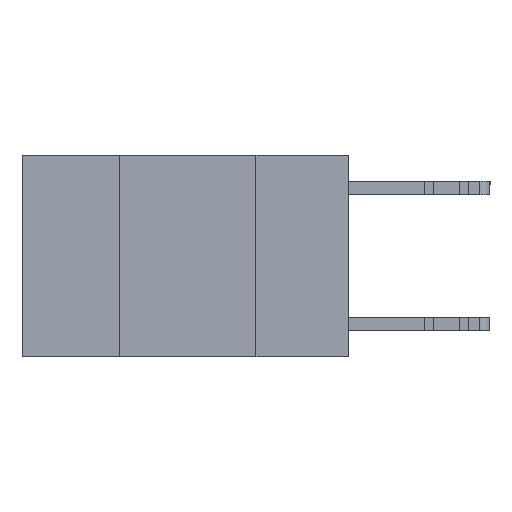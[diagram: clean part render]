
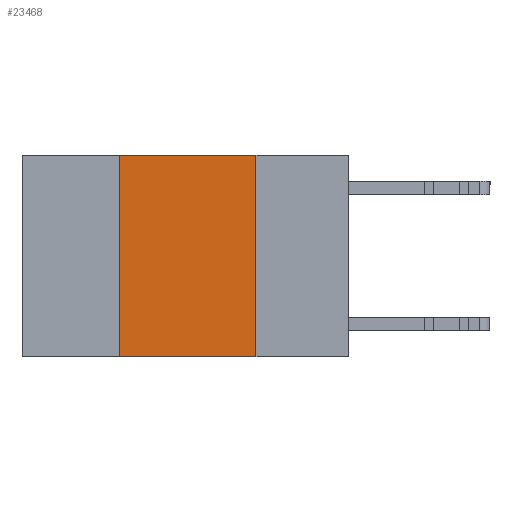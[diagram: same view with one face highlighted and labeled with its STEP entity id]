
A CAD part, left-side view. The second image highlights one B-rep face of the part: STEP entity #23468.
In plain terms, the highlighted planar face has unit normal (-1, 0, 0).
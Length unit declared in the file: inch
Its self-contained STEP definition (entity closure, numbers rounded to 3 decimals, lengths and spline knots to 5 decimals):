
#216 = ORIENTED_EDGE ( 'NONE', *, *, #1271, .F. ) ;
#508 = FACE_OUTER_BOUND ( 'NONE', #2229, .T. ) ;
#1271 = EDGE_CURVE ( 'NONE', #9255, #15199, #19150, .T. ) ;
#1525 = ORIENTED_EDGE ( 'NONE', *, *, #2031, .F. ) ;
#2031 = EDGE_CURVE ( 'NONE', #8859, #9255, #31517, .T. ) ;
#2229 = EDGE_LOOP ( 'NONE', ( #216, #1525, #17366, #27733 ) ) ;
#2416 = CARTESIAN_POINT ( 'NONE',  ( 0., 0.6, -0.37 ) ) ;
#2518 = CARTESIAN_POINT ( 'NONE',  ( 0., 0.17, 0. ) ) ;
#2830 = AXIS2_PLACEMENT_3D ( 'NONE', #25759, #25920, #25430 ) ;
#5098 = VECTOR ( 'NONE', #20353, 39.37008 ) ;
#6986 = VECTOR ( 'NONE', #31164, 39.37008 ) ;
#7247 = LINE ( 'NONE', #14903, #5098 ) ;
#8859 = VERTEX_POINT ( 'NONE', #17838 ) ;
#9255 = VERTEX_POINT ( 'NONE', #2518 ) ;
#14606 = VECTOR ( 'NONE', #21358, 39.37008 ) ;
#14903 = CARTESIAN_POINT ( 'NONE',  ( 0., 0.42, 0. ) ) ;
#15199 = VERTEX_POINT ( 'NONE', #25071 ) ;
#15637 = PLANE ( 'NONE',  #2830 ) ;
#17366 = ORIENTED_EDGE ( 'NONE', *, *, #25833, .F. ) ;
#17838 = CARTESIAN_POINT ( 'NONE',  ( 0., 0.42, 0. ) ) ;
#19150 = LINE ( 'NONE', #24146, #26186 ) ;
#20353 = DIRECTION ( 'NONE',  ( 0., 0., 1. ) ) ;
#20676 = LINE ( 'NONE', #2416, #6986 ) ;
#21358 = DIRECTION ( 'NONE',  ( 0., -1., 0. ) ) ;
#21985 = EDGE_CURVE ( 'NONE', #24960, #15199, #20676, .T. ) ;
#23468 = ADVANCED_FACE ( 'NONE', ( #508 ), #15637, .F. ) ;
#24146 = CARTESIAN_POINT ( 'NONE',  ( 0., 0.17, 0. ) ) ;
#24960 = VERTEX_POINT ( 'NONE', #26754 ) ;
#25071 = CARTESIAN_POINT ( 'NONE',  ( 0., 0.17, -0.37 ) ) ;
#25430 = DIRECTION ( 'NONE',  ( 0., 0., -1. ) ) ;
#25759 = CARTESIAN_POINT ( 'NONE',  ( 0., 0.6, 0. ) ) ;
#25833 = EDGE_CURVE ( 'NONE', #24960, #8859, #7247, .T. ) ;
#25920 = DIRECTION ( 'NONE',  ( 1., 0., 0. ) ) ;
#26186 = VECTOR ( 'NONE', #31475, 39.37008 ) ;
#26754 = CARTESIAN_POINT ( 'NONE',  ( 0., 0.42, -0.37 ) ) ;
#27733 = ORIENTED_EDGE ( 'NONE', *, *, #21985, .T. ) ;
#28857 = CARTESIAN_POINT ( 'NONE',  ( 0., 0.6, 0. ) ) ;
#31164 = DIRECTION ( 'NONE',  ( 0., -1., 0. ) ) ;
#31475 = DIRECTION ( 'NONE',  ( 0., 0., -1. ) ) ;
#31517 = LINE ( 'NONE', #28857, #14606 ) ;
